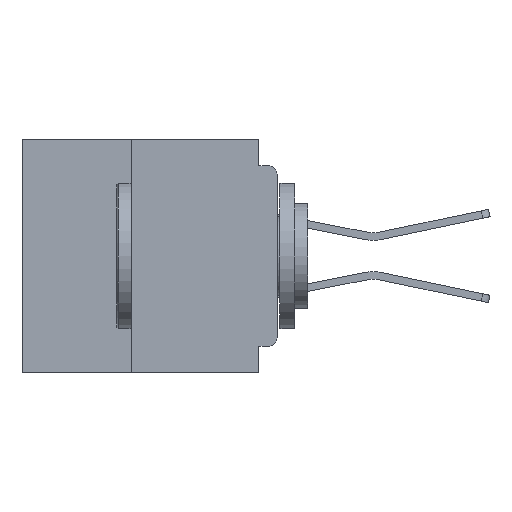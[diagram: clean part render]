
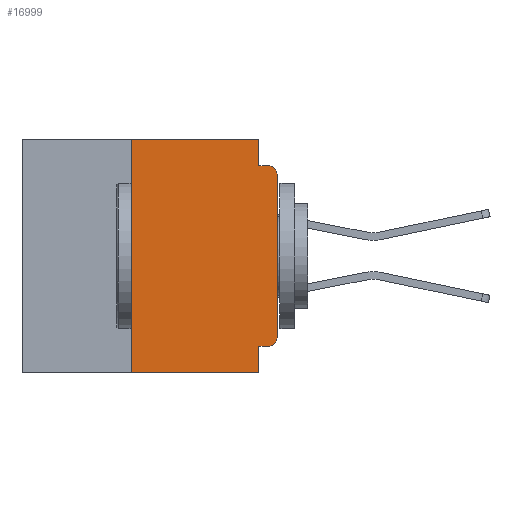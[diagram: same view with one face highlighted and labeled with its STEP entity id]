
A CAD part, left-side view. The second image highlights one B-rep face of the part: STEP entity #16999.
In plain terms, the highlighted planar face has unit normal (-1, 0, 0).
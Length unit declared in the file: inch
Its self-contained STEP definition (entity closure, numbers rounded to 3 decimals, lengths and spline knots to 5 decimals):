
#553 = AXIS2_PLACEMENT_3D ( 'NONE', #2847, #26881, #6357 ) ;
#984 = DIRECTION ( 'NONE',  ( -1., 0., 0. ) ) ;
#1057 = ORIENTED_EDGE ( 'NONE', *, *, #7262, .F. ) ;
#1472 = CARTESIAN_POINT ( 'NONE',  ( 0., 0.015, -0.355 ) ) ;
#1668 = EDGE_CURVE ( 'NONE', #34999, #38574, #41046, .T. ) ;
#1933 = DIRECTION ( 'NONE',  ( 0., -1., 0. ) ) ;
#1974 = CIRCLE ( 'NONE', #553, 0.015 ) ;
#2454 = CIRCLE ( 'NONE', #17486, 0.015 ) ;
#2841 = CARTESIAN_POINT ( 'NONE',  ( 0., 0.437, 0. ) ) ;
#2847 = CARTESIAN_POINT ( 'NONE',  ( 0., 0.015, -0.34 ) ) ;
#3203 = CARTESIAN_POINT ( 'NONE',  ( 0., 0.25, -0.4 ) ) ;
#3532 = CARTESIAN_POINT ( 'NONE',  ( 0., 0.437, 0. ) ) ;
#4067 = VERTEX_POINT ( 'NONE', #18410 ) ;
#4638 = VERTEX_POINT ( 'NONE', #1472 ) ;
#5432 = CARTESIAN_POINT ( 'NONE',  ( 0., 0., -0.045 ) ) ;
#5857 = DIRECTION ( 'NONE',  ( 0., 0., 1. ) ) ;
#6348 = DIRECTION ( 'NONE',  ( 0., 0., -1. ) ) ;
#6357 = DIRECTION ( 'NONE',  ( 0., 0., -1. ) ) ;
#6594 = ORIENTED_EDGE ( 'NONE', *, *, #7726, .F. ) ;
#6827 = LINE ( 'NONE', #13502, #42237 ) ;
#7262 = EDGE_CURVE ( 'NONE', #4638, #4067, #20707, .T. ) ;
#7726 = EDGE_CURVE ( 'NONE', #38574, #43834, #27629, .T. ) ;
#9135 = FACE_OUTER_BOUND ( 'NONE', #43928, .T. ) ;
#10313 = CARTESIAN_POINT ( 'NONE',  ( 0., 0.031, 0. ) ) ;
#11325 = AXIS2_PLACEMENT_3D ( 'NONE', #2841, #26876, #6348 ) ;
#11471 = CARTESIAN_POINT ( 'NONE',  ( 0., 0.031, -0.045 ) ) ;
#13122 = CARTESIAN_POINT ( 'NONE',  ( 0., 0.25, -0.4 ) ) ;
#13502 = CARTESIAN_POINT ( 'NONE',  ( 0., 0.031, -0.4 ) ) ;
#14559 = ORIENTED_EDGE ( 'NONE', *, *, #1668, .F. ) ;
#15004 = CARTESIAN_POINT ( 'NONE',  ( 0., 0., -0.355 ) ) ;
#15190 = VECTOR ( 'NONE', #36181, 39.37008 ) ;
#15875 = ORIENTED_EDGE ( 'NONE', *, *, #25619, .F. ) ;
#16999 = ADVANCED_FACE ( 'NONE', ( #9135 ), #30167, .F. ) ;
#17065 = EDGE_CURVE ( 'NONE', #34999, #23172, #42416, .T. ) ;
#17486 = AXIS2_PLACEMENT_3D ( 'NONE', #21609, #984, #25052 ) ;
#17739 = VECTOR ( 'NONE', #34312, 39.37008 ) ;
#18129 = VECTOR ( 'NONE', #1933, 39.37008 ) ;
#18410 = CARTESIAN_POINT ( 'NONE',  ( 0., 0.031, -0.355 ) ) ;
#18535 = VECTOR ( 'NONE', #37920, 39.37008 ) ;
#18628 = VERTEX_POINT ( 'NONE', #11471 ) ;
#19857 = ORIENTED_EDGE ( 'NONE', *, *, #43630, .T. ) ;
#20297 = CARTESIAN_POINT ( 'NONE',  ( 0., 0.437, -0.4 ) ) ;
#20401 = EDGE_CURVE ( 'NONE', #4638, #20769, #1974, .T. ) ;
#20707 = LINE ( 'NONE', #15004, #21795 ) ;
#20769 = VERTEX_POINT ( 'NONE', #32420 ) ;
#20975 = EDGE_CURVE ( 'NONE', #4067, #23172, #6827, .T. ) ;
#21609 = CARTESIAN_POINT ( 'NONE',  ( 0., 0.015, -0.06 ) ) ;
#21744 = VECTOR ( 'NONE', #5857, 39.37008 ) ;
#21795 = VECTOR ( 'NONE', #39037, 39.37008 ) ;
#22395 = CARTESIAN_POINT ( 'NONE',  ( 0., 0., 0. ) ) ;
#23172 = VERTEX_POINT ( 'NONE', #42601 ) ;
#23719 = DIRECTION ( 'NONE',  ( 0., -1., 0. ) ) ;
#24081 = EDGE_CURVE ( 'NONE', #43834, #18628, #26818, .T. ) ;
#25052 = DIRECTION ( 'NONE',  ( 0., 0., -1. ) ) ;
#25619 = EDGE_CURVE ( 'NONE', #18628, #36291, #37423, .T. ) ;
#26417 = CARTESIAN_POINT ( 'NONE',  ( 0., 0.25, 0. ) ) ;
#26818 = LINE ( 'NONE', #10313, #17739 ) ;
#26876 = DIRECTION ( 'NONE',  ( 1., 0., 0. ) ) ;
#26881 = DIRECTION ( 'NONE',  ( -1., 0., 0. ) ) ;
#27152 = VERTEX_POINT ( 'NONE', #34435 ) ;
#27629 = LINE ( 'NONE', #3532, #18535 ) ;
#30167 = PLANE ( 'NONE',  #11325 ) ;
#30360 = ORIENTED_EDGE ( 'NONE', *, *, #30914, .T. ) ;
#30914 = EDGE_CURVE ( 'NONE', #20769, #27152, #41514, .T. ) ;
#32420 = CARTESIAN_POINT ( 'NONE',  ( 0., 0., -0.34 ) ) ;
#33280 = VECTOR ( 'NONE', #23719, 39.37008 ) ;
#34070 = DIRECTION ( 'NONE',  ( 0., 0., -1. ) ) ;
#34312 = DIRECTION ( 'NONE',  ( 0., 0., -1. ) ) ;
#34435 = CARTESIAN_POINT ( 'NONE',  ( 0., 0., -0.06 ) ) ;
#34999 = VERTEX_POINT ( 'NONE', #13122 ) ;
#35902 = ORIENTED_EDGE ( 'NONE', *, *, #17065, .T. ) ;
#36181 = DIRECTION ( 'NONE',  ( 0., 0., 1. ) ) ;
#36291 = VERTEX_POINT ( 'NONE', #40766 ) ;
#37423 = LINE ( 'NONE', #5432, #18129 ) ;
#37920 = DIRECTION ( 'NONE',  ( 0., -1., 0. ) ) ;
#38467 = ORIENTED_EDGE ( 'NONE', *, *, #24081, .F. ) ;
#38574 = VERTEX_POINT ( 'NONE', #26417 ) ;
#39037 = DIRECTION ( 'NONE',  ( 0., 1., 0. ) ) ;
#39306 = ORIENTED_EDGE ( 'NONE', *, *, #20975, .F. ) ;
#39747 = CARTESIAN_POINT ( 'NONE',  ( 0., 0.031, 0. ) ) ;
#40766 = CARTESIAN_POINT ( 'NONE',  ( 0., 0.015, -0.045 ) ) ;
#41046 = LINE ( 'NONE', #3203, #21744 ) ;
#41514 = LINE ( 'NONE', #22395, #15190 ) ;
#42237 = VECTOR ( 'NONE', #34070, 39.37008 ) ;
#42416 = LINE ( 'NONE', #20297, #33280 ) ;
#42601 = CARTESIAN_POINT ( 'NONE',  ( 0., 0.031, -0.4 ) ) ;
#42655 = ORIENTED_EDGE ( 'NONE', *, *, #20401, .T. ) ;
#43630 = EDGE_CURVE ( 'NONE', #27152, #36291, #2454, .T. ) ;
#43834 = VERTEX_POINT ( 'NONE', #39747 ) ;
#43928 = EDGE_LOOP ( 'NONE', ( #30360, #19857, #15875, #38467, #6594, #14559, #35902, #39306, #1057, #42655 ) ) ;
